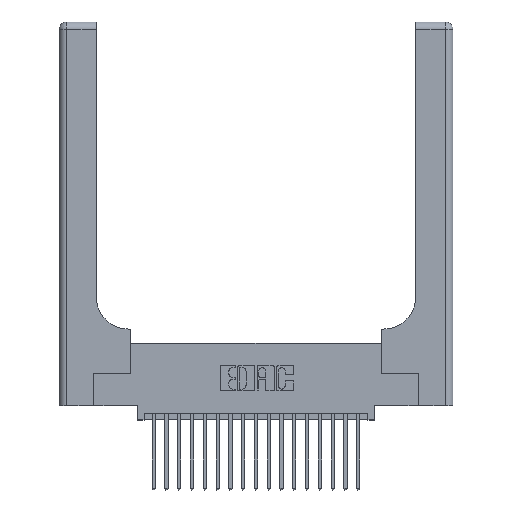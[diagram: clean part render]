
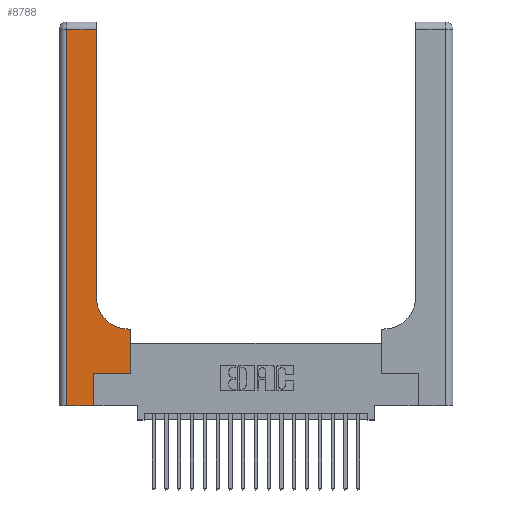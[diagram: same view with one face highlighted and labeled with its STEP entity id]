
A CAD part, top view. The second image highlights one B-rep face of the part: STEP entity #8788.
In plain terms, the highlighted planar face has unit normal (0, 0, 1).
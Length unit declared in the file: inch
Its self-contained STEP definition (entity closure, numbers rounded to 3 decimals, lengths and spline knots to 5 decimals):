
#113 = VECTOR ( 'NONE', #4357, 39.37008 ) ;
#309 = CARTESIAN_POINT ( 'NONE',  ( 0.2915, 3., 0.37 ) ) ;
#377 = VERTEX_POINT ( 'NONE', #9080 ) ;
#624 = CARTESIAN_POINT ( 'NONE',  ( 0.2915, 0.6, 0.37 ) ) ;
#626 = VERTEX_POINT ( 'NONE', #14189 ) ;
#744 = LINE ( 'NONE', #2939, #8471 ) ;
#1401 = DIRECTION ( 'NONE',  ( 0., 0., -1. ) ) ;
#1968 = VECTOR ( 'NONE', #6142, 39.37008 ) ;
#1973 = LINE ( 'NONE', #16318, #113 ) ;
#2072 = DIRECTION ( 'NONE',  ( 0., 1., 0. ) ) ;
#2893 = LINE ( 'NONE', #20673, #3673 ) ;
#2939 = CARTESIAN_POINT ( 'NONE',  ( 0., 0., 0.37 ) ) ;
#3673 = VECTOR ( 'NONE', #19276, 39.37008 ) ;
#3784 = AXIS2_PLACEMENT_3D ( 'NONE', #9875, #1401, #14995 ) ;
#4183 = CARTESIAN_POINT ( 'NONE',  ( 0.5585, 0.6, 0.37 ) ) ;
#4212 = EDGE_CURVE ( 'NONE', #17024, #7952, #744, .T. ) ;
#4357 = DIRECTION ( 'NONE',  ( -1., 0., 0. ) ) ;
#4460 = EDGE_CURVE ( 'NONE', #12831, #626, #12456, .T. ) ;
#4576 = ORIENTED_EDGE ( 'NONE', *, *, #10280, .T. ) ;
#5439 = LINE ( 'NONE', #17956, #1968 ) ;
#5504 = DIRECTION ( 'NONE',  ( 0., 1., 0. ) ) ;
#5884 = ORIENTED_EDGE ( 'NONE', *, *, #16292, .T. ) ;
#5965 = EDGE_CURVE ( 'NONE', #15924, #18497, #6267, .T. ) ;
#5990 = CARTESIAN_POINT ( 'NONE',  ( 0.5585, 0.25, 0.37 ) ) ;
#6142 = DIRECTION ( 'NONE',  ( 0., 1., 0. ) ) ;
#6267 = LINE ( 'NONE', #624, #9460 ) ;
#6321 = DIRECTION ( 'NONE',  ( 0., 0., -1. ) ) ;
#7572 = DIRECTION ( 'NONE',  ( -1., 0., 0. ) ) ;
#7678 = EDGE_CURVE ( 'NONE', #7952, #15217, #17356, .T. ) ;
#7952 = VERTEX_POINT ( 'NONE', #12100 ) ;
#8471 = VECTOR ( 'NONE', #14972, 39.37008 ) ;
#8764 = CARTESIAN_POINT ( 'NONE',  ( 0.269, 0.25, 0.37 ) ) ;
#8788 = ADVANCED_FACE ( 'NONE', ( #18643 ), #14991, .F. ) ;
#9080 = CARTESIAN_POINT ( 'NONE',  ( 0.06, 2.94, 0.37 ) ) ;
#9458 = ORIENTED_EDGE ( 'NONE', *, *, #5965, .T. ) ;
#9460 = VECTOR ( 'NONE', #7572, 39.37008 ) ;
#9781 = EDGE_CURVE ( 'NONE', #18497, #12831, #17299, .T. ) ;
#9875 = CARTESIAN_POINT ( 'NONE',  ( 0.5415, 0.85, 0.37 ) ) ;
#10280 = EDGE_CURVE ( 'NONE', #15237, #15924, #5439, .T. ) ;
#10333 = ORIENTED_EDGE ( 'NONE', *, *, #4460, .T. ) ;
#10884 = AXIS2_PLACEMENT_3D ( 'NONE', #11666, #6321, #18424 ) ;
#11294 = ORIENTED_EDGE ( 'NONE', *, *, #16864, .T. ) ;
#11666 = CARTESIAN_POINT ( 'NONE',  ( 0., 3., 0.37 ) ) ;
#12100 = CARTESIAN_POINT ( 'NONE',  ( 0.269, 0., 0.37 ) ) ;
#12111 = CARTESIAN_POINT ( 'NONE',  ( 0.5415, 0.6, 0.37 ) ) ;
#12456 = LINE ( 'NONE', #309, #21492 ) ;
#12514 = CARTESIAN_POINT ( 'NONE',  ( 0.269, 0., 0.37 ) ) ;
#12831 = VERTEX_POINT ( 'NONE', #18382 ) ;
#13489 = CARTESIAN_POINT ( 'NONE',  ( 0.06, 0., 0.37 ) ) ;
#13892 = VECTOR ( 'NONE', #2072, 39.37008 ) ;
#14189 = CARTESIAN_POINT ( 'NONE',  ( 0.2915, 2.94, 0.37 ) ) ;
#14273 = ORIENTED_EDGE ( 'NONE', *, *, #19591, .T. ) ;
#14488 = ORIENTED_EDGE ( 'NONE', *, *, #7678, .T. ) ;
#14537 = CARTESIAN_POINT ( 'NONE',  ( 0.269, 0.25, 0.37 ) ) ;
#14820 = ORIENTED_EDGE ( 'NONE', *, *, #4212, .T. ) ;
#14972 = DIRECTION ( 'NONE',  ( 1., 0., 0. ) ) ;
#14991 = PLANE ( 'NONE',  #10884 ) ;
#14995 = DIRECTION ( 'NONE',  ( 1., 0., 0. ) ) ;
#15217 = VERTEX_POINT ( 'NONE', #14537 ) ;
#15237 = VERTEX_POINT ( 'NONE', #5990 ) ;
#15924 = VERTEX_POINT ( 'NONE', #4183 ) ;
#16292 = EDGE_CURVE ( 'NONE', #15217, #15237, #21977, .T. ) ;
#16318 = CARTESIAN_POINT ( 'NONE',  ( 0., 2.94, 0.37 ) ) ;
#16864 = EDGE_CURVE ( 'NONE', #626, #377, #1973, .T. ) ;
#17024 = VERTEX_POINT ( 'NONE', #13489 ) ;
#17299 = CIRCLE ( 'NONE', #3784, 0.25 ) ;
#17356 = LINE ( 'NONE', #12514, #13892 ) ;
#17443 = VECTOR ( 'NONE', #20655, 39.37008 ) ;
#17636 = EDGE_LOOP ( 'NONE', ( #10333, #11294, #14273, #14820, #14488, #5884, #4576, #9458, #20256 ) ) ;
#17956 = CARTESIAN_POINT ( 'NONE',  ( 0.5585, 0.25, 0.37 ) ) ;
#18382 = CARTESIAN_POINT ( 'NONE',  ( 0.2915, 0.85, 0.37 ) ) ;
#18424 = DIRECTION ( 'NONE',  ( -1., 0., 0. ) ) ;
#18497 = VERTEX_POINT ( 'NONE', #12111 ) ;
#18643 = FACE_OUTER_BOUND ( 'NONE', #17636, .T. ) ;
#19276 = DIRECTION ( 'NONE',  ( 0., -1., 0. ) ) ;
#19591 = EDGE_CURVE ( 'NONE', #377, #17024, #2893, .T. ) ;
#20256 = ORIENTED_EDGE ( 'NONE', *, *, #9781, .T. ) ;
#20655 = DIRECTION ( 'NONE',  ( 1., 0., 0. ) ) ;
#20673 = CARTESIAN_POINT ( 'NONE',  ( 0.06, 3., 0.37 ) ) ;
#21492 = VECTOR ( 'NONE', #5504, 39.37008 ) ;
#21977 = LINE ( 'NONE', #8764, #17443 ) ;
